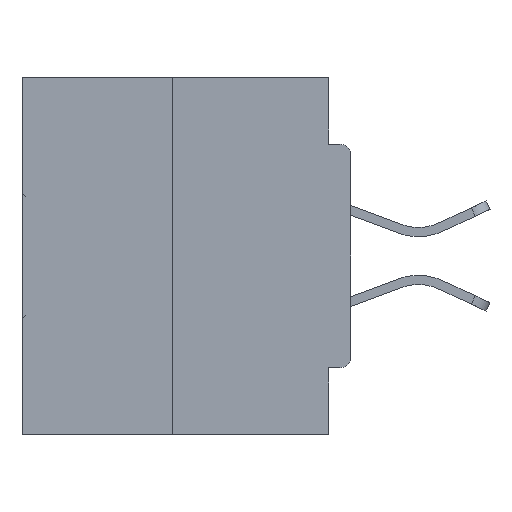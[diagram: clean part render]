
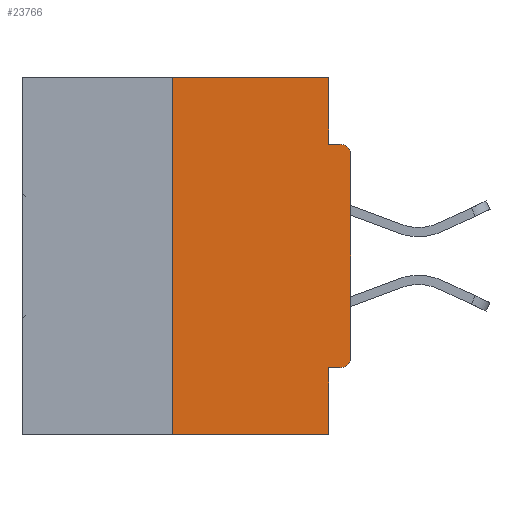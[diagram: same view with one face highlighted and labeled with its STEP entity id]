
A CAD part, left-side view. The second image highlights one B-rep face of the part: STEP entity #23766.
In plain terms, the highlighted planar face has unit normal (-1, 0, 0).
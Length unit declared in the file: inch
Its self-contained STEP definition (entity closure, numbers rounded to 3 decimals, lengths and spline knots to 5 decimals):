
#128 = LINE ( 'NONE', #14037, #44097 ) ;
#135 = LINE ( 'NONE', #14081, #8784 ) ;
#251 = LINE ( 'NONE', #22445, #14352 ) ;
#338 = CARTESIAN_POINT ( 'NONE',  ( 0., 0., -0.4065 ) ) ;
#1124 = FACE_OUTER_BOUND ( 'NONE', #1961, .T. ) ;
#1553 = CARTESIAN_POINT ( 'NONE',  ( 0., 0.031, 0. ) ) ;
#1961 = EDGE_LOOP ( 'NONE', ( #35883, #29851, #23563, #35266, #10990, #7591, #43589, #21735, #40258, #5740 ) ) ;
#2584 = CARTESIAN_POINT ( 'NONE',  ( 0., 0.46, 0. ) ) ;
#2724 = EDGE_CURVE ( 'NONE', #40587, #42162, #15960, .T. ) ;
#2813 = EDGE_CURVE ( 'NONE', #7504, #17070, #251, .T. ) ;
#3171 = DIRECTION ( 'NONE',  ( 0., 0., -1. ) ) ;
#3997 = DIRECTION ( 'NONE',  ( 0., 0., -1. ) ) ;
#4091 = CIRCLE ( 'NONE', #21961, 0.015 ) ;
#4842 = LINE ( 'NONE', #8085, #38499 ) ;
#4909 = VERTEX_POINT ( 'NONE', #26862 ) ;
#5130 = EDGE_CURVE ( 'NONE', #42162, #4909, #25561, .T. ) ;
#5740 = ORIENTED_EDGE ( 'NONE', *, *, #2813, .F. ) ;
#6217 = EDGE_CURVE ( 'NONE', #17070, #27605, #19469, .T. ) ;
#7504 = VERTEX_POINT ( 'NONE', #1553 ) ;
#7591 = ORIENTED_EDGE ( 'NONE', *, *, #43606, .T. ) ;
#8085 = CARTESIAN_POINT ( 'NONE',  ( 0., 0.46, -0.5 ) ) ;
#8784 = VECTOR ( 'NONE', #17421, 39.37008 ) ;
#9950 = EDGE_CURVE ( 'NONE', #39534, #4909, #4842, .T. ) ;
#10990 = ORIENTED_EDGE ( 'NONE', *, *, #2724, .F. ) ;
#11114 = DIRECTION ( 'NONE',  ( 0., -1., 0. ) ) ;
#11338 = VECTOR ( 'NONE', #12560, 39.37008 ) ;
#12560 = DIRECTION ( 'NONE',  ( 0., -1., 0. ) ) ;
#13338 = CARTESIAN_POINT ( 'NONE',  ( 0., 0.25, -0.5 ) ) ;
#13719 = EDGE_CURVE ( 'NONE', #39534, #25808, #135, .T. ) ;
#14037 = CARTESIAN_POINT ( 'NONE',  ( 0., 0., 0. ) ) ;
#14081 = CARTESIAN_POINT ( 'NONE',  ( 0., 0.25, 0. ) ) ;
#14352 = VECTOR ( 'NONE', #35815, 39.37008 ) ;
#14434 = DIRECTION ( 'NONE',  ( 0., 1., 0. ) ) ;
#15912 = DIRECTION ( 'NONE',  ( 0., 0., -1. ) ) ;
#15958 = CARTESIAN_POINT ( 'NONE',  ( 0., 0.031, -0.0935 ) ) ;
#15960 = LINE ( 'NONE', #338, #21960 ) ;
#16804 = DIRECTION ( 'NONE',  ( 0., -1., 0. ) ) ;
#17070 = VERTEX_POINT ( 'NONE', #15958 ) ;
#17421 = DIRECTION ( 'NONE',  ( 0., 0., 1. ) ) ;
#17665 = CIRCLE ( 'NONE', #24937, 0.015 ) ;
#17762 = CARTESIAN_POINT ( 'NONE',  ( 0., 0.015, -0.4065 ) ) ;
#19253 = DIRECTION ( 'NONE',  ( 1., 0., 0. ) ) ;
#19469 = LINE ( 'NONE', #22752, #11338 ) ;
#19838 = PLANE ( 'NONE',  #35184 ) ;
#19902 = EDGE_CURVE ( 'NONE', #25808, #7504, #41015, .T. ) ;
#20394 = CARTESIAN_POINT ( 'NONE',  ( 0., 0., -0.3915 ) ) ;
#21735 = ORIENTED_EDGE ( 'NONE', *, *, #35500, .T. ) ;
#21960 = VECTOR ( 'NONE', #14434, 39.37008 ) ;
#21961 = AXIS2_PLACEMENT_3D ( 'NONE', #27231, #27548, #3171 ) ;
#22445 = CARTESIAN_POINT ( 'NONE',  ( 0., 0.031, 0. ) ) ;
#22594 = DIRECTION ( 'NONE',  ( 0., 0., -1. ) ) ;
#22752 = CARTESIAN_POINT ( 'NONE',  ( 0., 0., -0.0935 ) ) ;
#23563 = ORIENTED_EDGE ( 'NONE', *, *, #9950, .T. ) ;
#23766 = ADVANCED_FACE ( 'NONE', ( #1124 ), #19838, .F. ) ;
#24748 = CARTESIAN_POINT ( 'NONE',  ( 0., 0.031, -0.5 ) ) ;
#24937 = AXIS2_PLACEMENT_3D ( 'NONE', #32445, #39923, #22594 ) ;
#25107 = CARTESIAN_POINT ( 'NONE',  ( 0., 0.25, 0. ) ) ;
#25561 = LINE ( 'NONE', #24748, #38671 ) ;
#25808 = VERTEX_POINT ( 'NONE', #25107 ) ;
#25851 = CARTESIAN_POINT ( 'NONE',  ( 0., 0., -0.1085 ) ) ;
#25937 = VERTEX_POINT ( 'NONE', #25851 ) ;
#26862 = CARTESIAN_POINT ( 'NONE',  ( 0., 0.031, -0.5 ) ) ;
#27231 = CARTESIAN_POINT ( 'NONE',  ( 0., 0.015, -0.3915 ) ) ;
#27548 = DIRECTION ( 'NONE',  ( -1., 0., 0. ) ) ;
#27605 = VERTEX_POINT ( 'NONE', #41066 ) ;
#29317 = EDGE_CURVE ( 'NONE', #39745, #25937, #128, .T. ) ;
#29851 = ORIENTED_EDGE ( 'NONE', *, *, #13719, .F. ) ;
#31749 = VECTOR ( 'NONE', #16804, 39.37008 ) ;
#32445 = CARTESIAN_POINT ( 'NONE',  ( 0., 0.015, -0.1085 ) ) ;
#35184 = AXIS2_PLACEMENT_3D ( 'NONE', #40090, #19253, #15912 ) ;
#35266 = ORIENTED_EDGE ( 'NONE', *, *, #5130, .F. ) ;
#35500 = EDGE_CURVE ( 'NONE', #25937, #27605, #17665, .T. ) ;
#35815 = DIRECTION ( 'NONE',  ( 0., 0., -1. ) ) ;
#35883 = ORIENTED_EDGE ( 'NONE', *, *, #19902, .F. ) ;
#38277 = DIRECTION ( 'NONE',  ( 0., 0., 1. ) ) ;
#38499 = VECTOR ( 'NONE', #11114, 39.37008 ) ;
#38671 = VECTOR ( 'NONE', #3997, 39.37008 ) ;
#39534 = VERTEX_POINT ( 'NONE', #13338 ) ;
#39745 = VERTEX_POINT ( 'NONE', #20394 ) ;
#39923 = DIRECTION ( 'NONE',  ( -1., 0., 0. ) ) ;
#40090 = CARTESIAN_POINT ( 'NONE',  ( 0., 0.46, 0. ) ) ;
#40258 = ORIENTED_EDGE ( 'NONE', *, *, #6217, .F. ) ;
#40587 = VERTEX_POINT ( 'NONE', #17762 ) ;
#41015 = LINE ( 'NONE', #2584, #31749 ) ;
#41066 = CARTESIAN_POINT ( 'NONE',  ( 0., 0.015, -0.0935 ) ) ;
#41552 = CARTESIAN_POINT ( 'NONE',  ( 0., 0.031, -0.4065 ) ) ;
#42162 = VERTEX_POINT ( 'NONE', #41552 ) ;
#43589 = ORIENTED_EDGE ( 'NONE', *, *, #29317, .T. ) ;
#43606 = EDGE_CURVE ( 'NONE', #40587, #39745, #4091, .T. ) ;
#44097 = VECTOR ( 'NONE', #38277, 39.37008 ) ;
